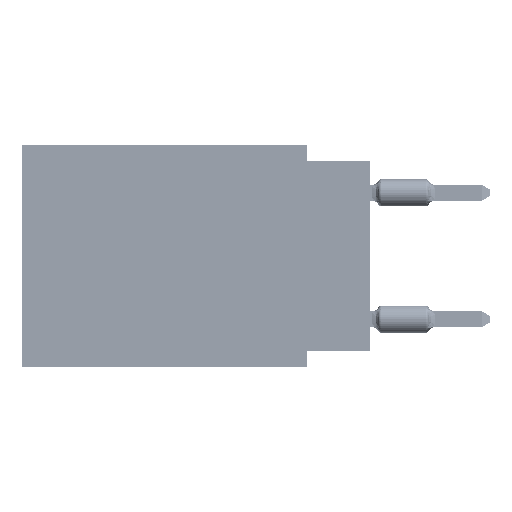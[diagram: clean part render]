
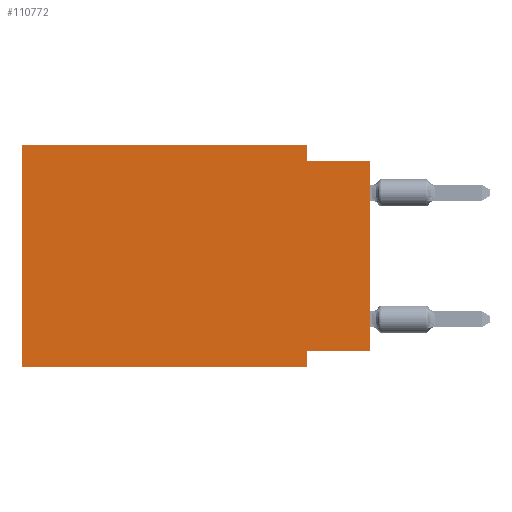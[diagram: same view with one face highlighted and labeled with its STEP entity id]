
A CAD part, left-side view. The second image highlights one B-rep face of the part: STEP entity #110772.
In plain terms, the highlighted planar face has unit normal (-1, 0, 0).
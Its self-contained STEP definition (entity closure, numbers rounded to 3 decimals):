
#6255 = VECTOR ( 'NONE', #57999, 1000. ) ;
#9044 = LINE ( 'NONE', #68104, #6255 ) ;
#11248 = EDGE_CURVE ( 'NONE', #83285, #52410, #37263, .T. ) ;
#12549 = EDGE_CURVE ( 'NONE', #14448, #47452, #58608, .T. ) ;
#13001 = DIRECTION ( 'NONE',  ( 0., 0., -1. ) ) ;
#14448 = VERTEX_POINT ( 'NONE', #35625 ) ;
#19168 = ORIENTED_EDGE ( 'NONE', *, *, #33783, .F. ) ;
#19513 = DIRECTION ( 'NONE',  ( 0., 0., -1. ) ) ;
#19616 = VECTOR ( 'NONE', #100826, 1000. ) ;
#20331 = PLANE ( 'NONE',  #80536 ) ;
#21307 = CARTESIAN_POINT ( 'NONE',  ( 0., 2.54, -0.635 ) ) ;
#24078 = ORIENTED_EDGE ( 'NONE', *, *, #11248, .F. ) ;
#26223 = LINE ( 'NONE', #61094, #58136 ) ;
#27497 = CARTESIAN_POINT ( 'NONE',  ( 0., 0., -8.255 ) ) ;
#27827 = VECTOR ( 'NONE', #109611, 1000. ) ;
#28068 = CARTESIAN_POINT ( 'NONE',  ( 0., 13.97, 0. ) ) ;
#28497 = CARTESIAN_POINT ( 'NONE',  ( 0., 2.54, -8.89 ) ) ;
#30530 = ORIENTED_EDGE ( 'NONE', *, *, #76854, .T. ) ;
#30672 = VECTOR ( 'NONE', #62381, 1000. ) ;
#31021 = DIRECTION ( 'NONE',  ( 0., 0., 1. ) ) ;
#31739 = VERTEX_POINT ( 'NONE', #82404 ) ;
#33783 = EDGE_CURVE ( 'NONE', #31739, #55026, #37506, .T. ) ;
#35625 = CARTESIAN_POINT ( 'NONE',  ( 0., 13.97, -8.89 ) ) ;
#37263 = LINE ( 'NONE', #63693, #89517 ) ;
#37506 = LINE ( 'NONE', #81955, #87065 ) ;
#40112 = EDGE_CURVE ( 'NONE', #51030, #50348, #57467, .T. ) ;
#42335 = ORIENTED_EDGE ( 'NONE', *, *, #40112, .T. ) ;
#46363 = VECTOR ( 'NONE', #31021, 1000. ) ;
#47155 = ORIENTED_EDGE ( 'NONE', *, *, #106748, .F. ) ;
#47452 = VERTEX_POINT ( 'NONE', #56629 ) ;
#50348 = VERTEX_POINT ( 'NONE', #74421 ) ;
#51030 = VERTEX_POINT ( 'NONE', #27497 ) ;
#51295 = ORIENTED_EDGE ( 'NONE', *, *, #77368, .F. ) ;
#52136 = ORIENTED_EDGE ( 'NONE', *, *, #84417, .F. ) ;
#52410 = VERTEX_POINT ( 'NONE', #21307 ) ;
#54267 = CARTESIAN_POINT ( 'NONE',  ( 0., 2.54, 0. ) ) ;
#54660 = CARTESIAN_POINT ( 'NONE',  ( 0., 13.97, 0. ) ) ;
#54711 = DIRECTION ( 'NONE',  ( 0., 0., -1. ) ) ;
#55026 = VERTEX_POINT ( 'NONE', #28497 ) ;
#56629 = CARTESIAN_POINT ( 'NONE',  ( 0., 13.97, 0. ) ) ;
#56888 = DIRECTION ( 'NONE',  ( 1., 0., 0. ) ) ;
#57467 = LINE ( 'NONE', #82248, #46363 ) ;
#57999 = DIRECTION ( 'NONE',  ( 0., -1., 0. ) ) ;
#58136 = VECTOR ( 'NONE', #110057, 1000. ) ;
#58608 = LINE ( 'NONE', #66484, #19616 ) ;
#61094 = CARTESIAN_POINT ( 'NONE',  ( 0., 0., -0.635 ) ) ;
#62381 = DIRECTION ( 'NONE',  ( 0., -1., 0. ) ) ;
#63693 = CARTESIAN_POINT ( 'NONE',  ( 0., 2.54, 0. ) ) ;
#66484 = CARTESIAN_POINT ( 'NONE',  ( 0., 13.97, 0. ) ) ;
#68104 = CARTESIAN_POINT ( 'NONE',  ( 0., 13.97, -8.89 ) ) ;
#74421 = CARTESIAN_POINT ( 'NONE',  ( 0., 0., -0.635 ) ) ;
#76854 = EDGE_CURVE ( 'NONE', #14448, #55026, #9044, .T. ) ;
#77368 = EDGE_CURVE ( 'NONE', #51030, #31739, #85982, .T. ) ;
#79654 = ORIENTED_EDGE ( 'NONE', *, *, #12549, .F. ) ;
#80536 = AXIS2_PLACEMENT_3D ( 'NONE', #54660, #56888, #13001 ) ;
#81955 = CARTESIAN_POINT ( 'NONE',  ( 0., 2.54, -8.89 ) ) ;
#82248 = CARTESIAN_POINT ( 'NONE',  ( 0., 0., 0. ) ) ;
#82404 = CARTESIAN_POINT ( 'NONE',  ( 0., 2.54, -8.255 ) ) ;
#83285 = VERTEX_POINT ( 'NONE', #54267 ) ;
#84417 = EDGE_CURVE ( 'NONE', #52410, #50348, #26223, .T. ) ;
#85982 = LINE ( 'NONE', #110155, #27827 ) ;
#87065 = VECTOR ( 'NONE', #19513, 1000. ) ;
#89517 = VECTOR ( 'NONE', #54711, 1000. ) ;
#90094 = FACE_OUTER_BOUND ( 'NONE', #110441, .T. ) ;
#100826 = DIRECTION ( 'NONE',  ( 0., 0., 1. ) ) ;
#106251 = LINE ( 'NONE', #28068, #30672 ) ;
#106748 = EDGE_CURVE ( 'NONE', #47452, #83285, #106251, .T. ) ;
#109611 = DIRECTION ( 'NONE',  ( 0., 1., 0. ) ) ;
#110057 = DIRECTION ( 'NONE',  ( 0., -1., 0. ) ) ;
#110155 = CARTESIAN_POINT ( 'NONE',  ( 0., 0., -8.255 ) ) ;
#110441 = EDGE_LOOP ( 'NONE', ( #42335, #52136, #24078, #47155, #79654, #30530, #19168, #51295 ) ) ;
#110772 = ADVANCED_FACE ( 'NONE', ( #90094 ), #20331, .F. ) ;
